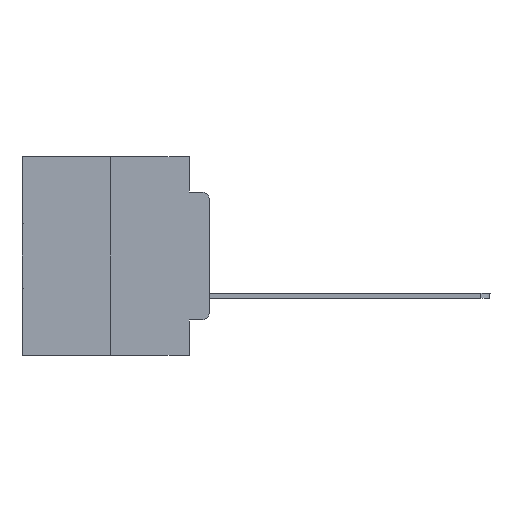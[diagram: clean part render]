
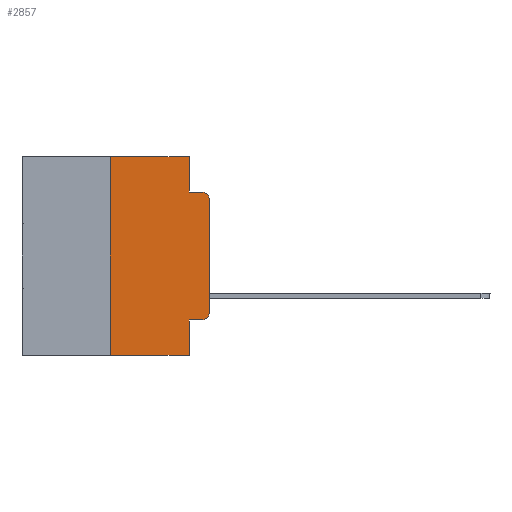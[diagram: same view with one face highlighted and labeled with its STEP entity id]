
A CAD part, left-side view. The second image highlights one B-rep face of the part: STEP entity #2857.
In plain terms, the highlighted planar face has unit normal (-1, 0, 0).
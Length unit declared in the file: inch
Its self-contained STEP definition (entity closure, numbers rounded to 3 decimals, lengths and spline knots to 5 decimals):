
#242 = LINE ( 'NONE', #18213, #20198 ) ;
#902 = DIRECTION ( 'NONE',  ( 0., 0., 1. ) ) ;
#1255 = ORIENTED_EDGE ( 'NONE', *, *, #22709, .F. ) ;
#1283 = VERTEX_POINT ( 'NONE', #10862 ) ;
#1286 = CARTESIAN_POINT ( 'NONE',  ( 0., 0.02, -0.4115 ) ) ;
#1892 = CIRCLE ( 'NONE', #5640, 0.02 ) ;
#2065 = VECTOR ( 'NONE', #17311, 39.37008 ) ;
#2857 = ADVANCED_FACE ( 'NONE', ( #16890 ), #15106, .F. ) ;
#3582 = VECTOR ( 'NONE', #26681, 39.37008 ) ;
#3857 = DIRECTION ( 'NONE',  ( 0., -1., 0. ) ) ;
#4211 = ORIENTED_EDGE ( 'NONE', *, *, #13587, .F. ) ;
#4835 = VECTOR ( 'NONE', #902, 39.37008 ) ;
#5058 = ORIENTED_EDGE ( 'NONE', *, *, #14664, .T. ) ;
#5440 = CARTESIAN_POINT ( 'NONE',  ( 0., 0.02, -0.1085 ) ) ;
#5640 = AXIS2_PLACEMENT_3D ( 'NONE', #17457, #19961, #12866 ) ;
#6129 = CARTESIAN_POINT ( 'NONE',  ( 0., 0.473, 0. ) ) ;
#6531 = VERTEX_POINT ( 'NONE', #24935 ) ;
#6561 = ORIENTED_EDGE ( 'NONE', *, *, #12848, .F. ) ;
#6661 = CARTESIAN_POINT ( 'NONE',  ( 0., 0.051, 0. ) ) ;
#7357 = DIRECTION ( 'NONE',  ( -1., 0., 0. ) ) ;
#7889 = ORIENTED_EDGE ( 'NONE', *, *, #13872, .T. ) ;
#8307 = CARTESIAN_POINT ( 'NONE',  ( 0., 0.051, -0.0885 ) ) ;
#8369 = VECTOR ( 'NONE', #18285, 39.37008 ) ;
#8395 = VECTOR ( 'NONE', #16235, 39.37008 ) ;
#8999 = VERTEX_POINT ( 'NONE', #1286 ) ;
#9278 = CARTESIAN_POINT ( 'NONE',  ( 0., 0.051, 0. ) ) ;
#10016 = CARTESIAN_POINT ( 'NONE',  ( 0., 0., 0. ) ) ;
#10245 = CIRCLE ( 'NONE', #18271, 0.02 ) ;
#10622 = CARTESIAN_POINT ( 'NONE',  ( 0., 0.473, -0.5 ) ) ;
#10862 = CARTESIAN_POINT ( 'NONE',  ( 0., 0.051, -0.0885 ) ) ;
#11813 = LINE ( 'NONE', #15644, #8395 ) ;
#12169 = VECTOR ( 'NONE', #3857, 39.37008 ) ;
#12715 = VERTEX_POINT ( 'NONE', #26654 ) ;
#12790 = EDGE_CURVE ( 'NONE', #6531, #22101, #15758, .T. ) ;
#12848 = EDGE_CURVE ( 'NONE', #12715, #15534, #28970, .T. ) ;
#12866 = DIRECTION ( 'NONE',  ( 0., 0., -1. ) ) ;
#12913 = EDGE_CURVE ( 'NONE', #28971, #27582, #10245, .T. ) ;
#13559 = LINE ( 'NONE', #6661, #3582 ) ;
#13587 = EDGE_CURVE ( 'NONE', #22101, #25445, #11813, .T. ) ;
#13681 = DIRECTION ( 'NONE',  ( 0., 0., 1. ) ) ;
#13872 = EDGE_CURVE ( 'NONE', #6531, #15534, #28838, .T. ) ;
#13939 = CARTESIAN_POINT ( 'NONE',  ( 0., 0., -0.3915 ) ) ;
#14421 = EDGE_CURVE ( 'NONE', #12715, #8999, #242, .T. ) ;
#14664 = EDGE_CURVE ( 'NONE', #8999, #16916, #1892, .T. ) ;
#15106 = PLANE ( 'NONE',  #19680 ) ;
#15534 = VERTEX_POINT ( 'NONE', #21639 ) ;
#15591 = ORIENTED_EDGE ( 'NONE', *, *, #12790, .F. ) ;
#15644 = CARTESIAN_POINT ( 'NONE',  ( 0., 0.473, 0. ) ) ;
#15758 = LINE ( 'NONE', #24582, #22467 ) ;
#16235 = DIRECTION ( 'NONE',  ( 0., -1., 0. ) ) ;
#16785 = DIRECTION ( 'NONE',  ( 0., 0., -1. ) ) ;
#16890 = FACE_OUTER_BOUND ( 'NONE', #21840, .T. ) ;
#16916 = VERTEX_POINT ( 'NONE', #13939 ) ;
#17311 = DIRECTION ( 'NONE',  ( 0., -1., 0. ) ) ;
#17457 = CARTESIAN_POINT ( 'NONE',  ( 0., 0.02, -0.3915 ) ) ;
#17607 = CARTESIAN_POINT ( 'NONE',  ( 0., 0., -0.1085 ) ) ;
#17815 = EDGE_CURVE ( 'NONE', #16916, #28971, #23562, .T. ) ;
#18213 = CARTESIAN_POINT ( 'NONE',  ( 0., 0.051, -0.4115 ) ) ;
#18271 = AXIS2_PLACEMENT_3D ( 'NONE', #5440, #7357, #16785 ) ;
#18285 = DIRECTION ( 'NONE',  ( 0., 0., -1. ) ) ;
#18336 = ORIENTED_EDGE ( 'NONE', *, *, #12913, .T. ) ;
#18945 = EDGE_CURVE ( 'NONE', #1283, #27582, #19667, .T. ) ;
#19667 = LINE ( 'NONE', #8307, #2065 ) ;
#19680 = AXIS2_PLACEMENT_3D ( 'NONE', #6129, #28330, #21437 ) ;
#19961 = DIRECTION ( 'NONE',  ( -1., 0., 0. ) ) ;
#20198 = VECTOR ( 'NONE', #20710, 39.37008 ) ;
#20710 = DIRECTION ( 'NONE',  ( 0., -1., 0. ) ) ;
#21437 = DIRECTION ( 'NONE',  ( 0., 0., -1. ) ) ;
#21639 = CARTESIAN_POINT ( 'NONE',  ( 0., 0.051, -0.5 ) ) ;
#21840 = EDGE_LOOP ( 'NONE', ( #23012, #18336, #26852, #1255, #4211, #15591, #7889, #6561, #24633, #5058 ) ) ;
#22101 = VERTEX_POINT ( 'NONE', #27361 ) ;
#22137 = CARTESIAN_POINT ( 'NONE',  ( 0., 0.02, -0.0885 ) ) ;
#22467 = VECTOR ( 'NONE', #13681, 39.37008 ) ;
#22709 = EDGE_CURVE ( 'NONE', #25445, #1283, #13559, .T. ) ;
#23012 = ORIENTED_EDGE ( 'NONE', *, *, #17815, .T. ) ;
#23562 = LINE ( 'NONE', #10016, #4835 ) ;
#24400 = CARTESIAN_POINT ( 'NONE',  ( 0., 0.051, 0. ) ) ;
#24582 = CARTESIAN_POINT ( 'NONE',  ( 0., 0.25, 0. ) ) ;
#24633 = ORIENTED_EDGE ( 'NONE', *, *, #14421, .T. ) ;
#24935 = CARTESIAN_POINT ( 'NONE',  ( 0., 0.25, -0.5 ) ) ;
#25445 = VERTEX_POINT ( 'NONE', #24400 ) ;
#26654 = CARTESIAN_POINT ( 'NONE',  ( 0., 0.051, -0.4115 ) ) ;
#26681 = DIRECTION ( 'NONE',  ( 0., 0., -1. ) ) ;
#26852 = ORIENTED_EDGE ( 'NONE', *, *, #18945, .F. ) ;
#27361 = CARTESIAN_POINT ( 'NONE',  ( 0., 0.25, 0. ) ) ;
#27582 = VERTEX_POINT ( 'NONE', #22137 ) ;
#28330 = DIRECTION ( 'NONE',  ( 1., 0., 0. ) ) ;
#28838 = LINE ( 'NONE', #10622, #12169 ) ;
#28970 = LINE ( 'NONE', #9278, #8369 ) ;
#28971 = VERTEX_POINT ( 'NONE', #17607 ) ;
